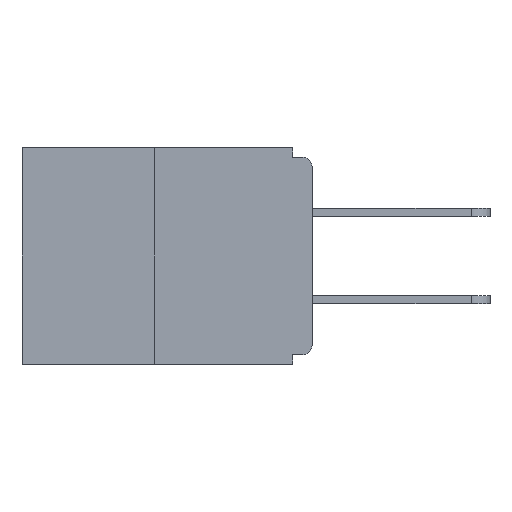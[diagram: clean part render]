
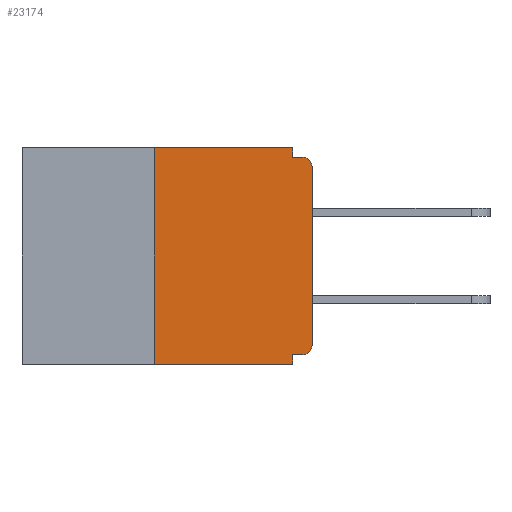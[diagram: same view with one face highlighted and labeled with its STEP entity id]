
A CAD part, left-side view. The second image highlights one B-rep face of the part: STEP entity #23174.
In plain terms, the highlighted planar face has unit normal (-1, 0, 0).
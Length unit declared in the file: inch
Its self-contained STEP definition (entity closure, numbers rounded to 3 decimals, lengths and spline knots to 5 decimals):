
#1280 = CARTESIAN_POINT ( 'NONE',  ( 0., 0.031, 0. ) ) ;
#1430 = AXIS2_PLACEMENT_3D ( 'NONE', #11281, #3889, #16280 ) ;
#2817 = CARTESIAN_POINT ( 'NONE',  ( 0., 0.25, 0. ) ) ;
#2946 = DIRECTION ( 'NONE',  ( -1., 0., 0. ) ) ;
#3381 = VERTEX_POINT ( 'NONE', #3942 ) ;
#3889 = DIRECTION ( 'NONE',  ( -1., 0., 0. ) ) ;
#3942 = CARTESIAN_POINT ( 'NONE',  ( 0., 0., -0.313 ) ) ;
#4236 = CARTESIAN_POINT ( 'NONE',  ( 0., 0.031, -0.328 ) ) ;
#4337 = VECTOR ( 'NONE', #9410, 39.37008 ) ;
#4385 = VERTEX_POINT ( 'NONE', #28847 ) ;
#4549 = VECTOR ( 'NONE', #7968, 39.37008 ) ;
#4689 = CARTESIAN_POINT ( 'NONE',  ( 0., 0.015, -0.015 ) ) ;
#5244 = VERTEX_POINT ( 'NONE', #4236 ) ;
#5283 = EDGE_CURVE ( 'NONE', #30398, #4385, #7406, .T. ) ;
#6280 = VERTEX_POINT ( 'NONE', #10504 ) ;
#6600 = EDGE_CURVE ( 'NONE', #30398, #27494, #18659, .T. ) ;
#7406 = LINE ( 'NONE', #2817, #28493 ) ;
#7844 = CIRCLE ( 'NONE', #30637, 0.015 ) ;
#7968 = DIRECTION ( 'NONE',  ( 0., 0., -1. ) ) ;
#8319 = VECTOR ( 'NONE', #26496, 39.37008 ) ;
#8349 = DIRECTION ( 'NONE',  ( 0., 0., -1. ) ) ;
#8574 = ORIENTED_EDGE ( 'NONE', *, *, #30459, .F. ) ;
#9410 = DIRECTION ( 'NONE',  ( 0., -1., 0. ) ) ;
#9477 = CARTESIAN_POINT ( 'NONE',  ( 0., 0.46, 0. ) ) ;
#9680 = CARTESIAN_POINT ( 'NONE',  ( 0., 0.031, -0.015 ) ) ;
#9683 = CARTESIAN_POINT ( 'NONE',  ( 0., 0., -0.015 ) ) ;
#9757 = VERTEX_POINT ( 'NONE', #1280 ) ;
#10174 = LINE ( 'NONE', #21861, #4337 ) ;
#10504 = CARTESIAN_POINT ( 'NONE',  ( 0., 0.015, -0.328 ) ) ;
#10581 = CARTESIAN_POINT ( 'NONE',  ( 0., 0.031, 0. ) ) ;
#10859 = VECTOR ( 'NONE', #29016, 39.37008 ) ;
#11065 = VERTEX_POINT ( 'NONE', #9680 ) ;
#11281 = CARTESIAN_POINT ( 'NONE',  ( 0., 0.015, -0.313 ) ) ;
#11406 = CIRCLE ( 'NONE', #1430, 0.015 ) ;
#11522 = CARTESIAN_POINT ( 'NONE',  ( 0., 0., -0.328 ) ) ;
#11878 = ORIENTED_EDGE ( 'NONE', *, *, #5283, .F. ) ;
#12049 = ORIENTED_EDGE ( 'NONE', *, *, #24884, .F. ) ;
#12093 = DIRECTION ( 'NONE',  ( 0., -1., 0. ) ) ;
#12299 = CARTESIAN_POINT ( 'NONE',  ( 0., 0.46, -0.343 ) ) ;
#12385 = DIRECTION ( 'NONE',  ( 0., 0., 1. ) ) ;
#12624 = CARTESIAN_POINT ( 'NONE',  ( 0., 0.031, -0.343 ) ) ;
#14092 = VECTOR ( 'NONE', #27608, 39.37008 ) ;
#14811 = DIRECTION ( 'NONE',  ( 0., -1., 0. ) ) ;
#16280 = DIRECTION ( 'NONE',  ( 0., 0., -1. ) ) ;
#17103 = ORIENTED_EDGE ( 'NONE', *, *, #19285, .T. ) ;
#18217 = LINE ( 'NONE', #10581, #4549 ) ;
#18308 = LINE ( 'NONE', #11522, #10859 ) ;
#18330 = ORIENTED_EDGE ( 'NONE', *, *, #31710, .F. ) ;
#18608 = ORIENTED_EDGE ( 'NONE', *, *, #30979, .F. ) ;
#18659 = LINE ( 'NONE', #12299, #22978 ) ;
#19048 = ORIENTED_EDGE ( 'NONE', *, *, #20580, .T. ) ;
#19285 = EDGE_CURVE ( 'NONE', #3381, #26514, #26701, .T. ) ;
#20580 = EDGE_CURVE ( 'NONE', #6280, #3381, #11406, .T. ) ;
#20990 = FACE_OUTER_BOUND ( 'NONE', #22995, .T. ) ;
#21449 = VERTEX_POINT ( 'NONE', #4689 ) ;
#21561 = ORIENTED_EDGE ( 'NONE', *, *, #27703, .T. ) ;
#21861 = CARTESIAN_POINT ( 'NONE',  ( 0., 0.46, 0. ) ) ;
#21932 = DIRECTION ( 'NONE',  ( 1., 0., 0. ) ) ;
#22978 = VECTOR ( 'NONE', #12093, 39.37008 ) ;
#22995 = EDGE_LOOP ( 'NONE', ( #18608, #11878, #25543, #26576, #8574, #19048, #17103, #21561, #18330, #12049 ) ) ;
#23174 = ADVANCED_FACE ( 'NONE', ( #20990 ), #26860, .F. ) ;
#23506 = CARTESIAN_POINT ( 'NONE',  ( 0., 0.031, -0.343 ) ) ;
#24884 = EDGE_CURVE ( 'NONE', #9757, #11065, #18217, .T. ) ;
#25543 = ORIENTED_EDGE ( 'NONE', *, *, #6600, .T. ) ;
#25648 = CARTESIAN_POINT ( 'NONE',  ( 0., 0.015, -0.03 ) ) ;
#25664 = LINE ( 'NONE', #9683, #29919 ) ;
#26496 = DIRECTION ( 'NONE',  ( 0., 0., 1. ) ) ;
#26514 = VERTEX_POINT ( 'NONE', #29487 ) ;
#26576 = ORIENTED_EDGE ( 'NONE', *, *, #27650, .F. ) ;
#26701 = LINE ( 'NONE', #28698, #8319 ) ;
#26860 = PLANE ( 'NONE',  #30344 ) ;
#27494 = VERTEX_POINT ( 'NONE', #23506 ) ;
#27608 = DIRECTION ( 'NONE',  ( 0., 0., -1. ) ) ;
#27650 = EDGE_CURVE ( 'NONE', #5244, #27494, #31303, .T. ) ;
#27703 = EDGE_CURVE ( 'NONE', #26514, #21449, #7844, .T. ) ;
#28493 = VECTOR ( 'NONE', #12385, 39.37008 ) ;
#28698 = CARTESIAN_POINT ( 'NONE',  ( 0., 0., 0. ) ) ;
#28847 = CARTESIAN_POINT ( 'NONE',  ( 0., 0.25, 0. ) ) ;
#29016 = DIRECTION ( 'NONE',  ( 0., 1., 0. ) ) ;
#29354 = DIRECTION ( 'NONE',  ( 0., 0., -1. ) ) ;
#29487 = CARTESIAN_POINT ( 'NONE',  ( 0., 0., -0.03 ) ) ;
#29919 = VECTOR ( 'NONE', #14811, 39.37008 ) ;
#30344 = AXIS2_PLACEMENT_3D ( 'NONE', #9477, #21932, #29354 ) ;
#30398 = VERTEX_POINT ( 'NONE', #31862 ) ;
#30459 = EDGE_CURVE ( 'NONE', #6280, #5244, #18308, .T. ) ;
#30637 = AXIS2_PLACEMENT_3D ( 'NONE', #25648, #2946, #8349 ) ;
#30979 = EDGE_CURVE ( 'NONE', #4385, #9757, #10174, .T. ) ;
#31303 = LINE ( 'NONE', #12624, #14092 ) ;
#31710 = EDGE_CURVE ( 'NONE', #11065, #21449, #25664, .T. ) ;
#31862 = CARTESIAN_POINT ( 'NONE',  ( 0., 0.25, -0.343 ) ) ;
